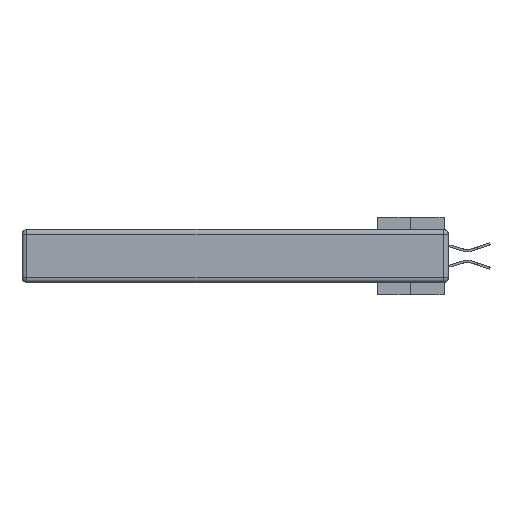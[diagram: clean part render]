
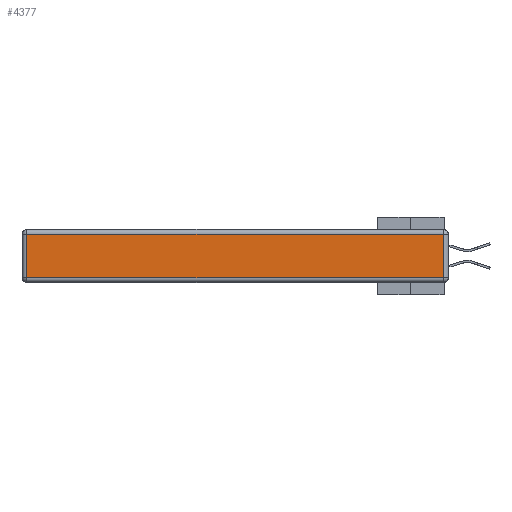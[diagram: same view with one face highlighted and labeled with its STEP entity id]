
A CAD part, left-side view. The second image highlights one B-rep face of the part: STEP entity #4377.
In plain terms, the highlighted planar face has unit normal (-1, 0, 0).
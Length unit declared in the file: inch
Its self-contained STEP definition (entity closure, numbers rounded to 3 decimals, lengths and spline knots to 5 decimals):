
#798 = EDGE_CURVE ( 'NONE', #42167, #6230, #36487, .T. ) ;
#918 = CARTESIAN_POINT ( 'NONE',  ( 0., 0., -0.343 ) ) ;
#1745 = CARTESIAN_POINT ( 'NONE',  ( 0., 2.72, -0.03 ) ) ;
#1755 = CARTESIAN_POINT ( 'NONE',  ( 0., 2.72, -0.343 ) ) ;
#4377 = ADVANCED_FACE ( 'NONE', ( #9529 ), #40044, .T. ) ;
#5097 = LINE ( 'NONE', #30043, #40217 ) ;
#5354 = EDGE_CURVE ( 'NONE', #11293, #42167, #21943, .T. ) ;
#6026 = LINE ( 'NONE', #22678, #25920 ) ;
#6230 = VERTEX_POINT ( 'NONE', #11808 ) ;
#7603 = DIRECTION ( 'NONE',  ( -1., 0., 0. ) ) ;
#7911 = DIRECTION ( 'NONE',  ( 0., 0., 1. ) ) ;
#9035 = DIRECTION ( 'NONE',  ( 0., 0., -1. ) ) ;
#9419 = CARTESIAN_POINT ( 'NONE',  ( 0., 0., -0.313 ) ) ;
#9529 = FACE_OUTER_BOUND ( 'NONE', #44506, .T. ) ;
#9908 = DIRECTION ( 'NONE',  ( 0., -1., 0. ) ) ;
#11293 = VERTEX_POINT ( 'NONE', #1745 ) ;
#11808 = CARTESIAN_POINT ( 'NONE',  ( 0., 0.03, -0.313 ) ) ;
#12884 = EDGE_CURVE ( 'NONE', #22142, #11293, #5097, .T. ) ;
#15138 = DIRECTION ( 'NONE',  ( 0., 0., 1. ) ) ;
#21943 = LINE ( 'NONE', #1755, #39451 ) ;
#22142 = VERTEX_POINT ( 'NONE', #24572 ) ;
#22678 = CARTESIAN_POINT ( 'NONE',  ( 0., 0.03, -0.343 ) ) ;
#22695 = ORIENTED_EDGE ( 'NONE', *, *, #12884, .T. ) ;
#23456 = VECTOR ( 'NONE', #9908, 39.37008 ) ;
#24572 = CARTESIAN_POINT ( 'NONE',  ( 0., 0.03, -0.03 ) ) ;
#25920 = VECTOR ( 'NONE', #15138, 39.37008 ) ;
#27974 = ORIENTED_EDGE ( 'NONE', *, *, #5354, .T. ) ;
#29472 = ORIENTED_EDGE ( 'NONE', *, *, #46527, .T. ) ;
#29730 = DIRECTION ( 'NONE',  ( 0., 1., 0. ) ) ;
#30043 = CARTESIAN_POINT ( 'NONE',  ( 0., 2.75, -0.03 ) ) ;
#32356 = ORIENTED_EDGE ( 'NONE', *, *, #798, .T. ) ;
#36487 = LINE ( 'NONE', #9419, #23456 ) ;
#39451 = VECTOR ( 'NONE', #9035, 39.37008 ) ;
#40044 = PLANE ( 'NONE',  #41029 ) ;
#40217 = VECTOR ( 'NONE', #29730, 39.37008 ) ;
#41029 = AXIS2_PLACEMENT_3D ( 'NONE', #918, #7603, #7911 ) ;
#42167 = VERTEX_POINT ( 'NONE', #43384 ) ;
#43384 = CARTESIAN_POINT ( 'NONE',  ( 0., 2.72, -0.313 ) ) ;
#44506 = EDGE_LOOP ( 'NONE', ( #32356, #29472, #22695, #27974 ) ) ;
#46527 = EDGE_CURVE ( 'NONE', #6230, #22142, #6026, .T. ) ;
